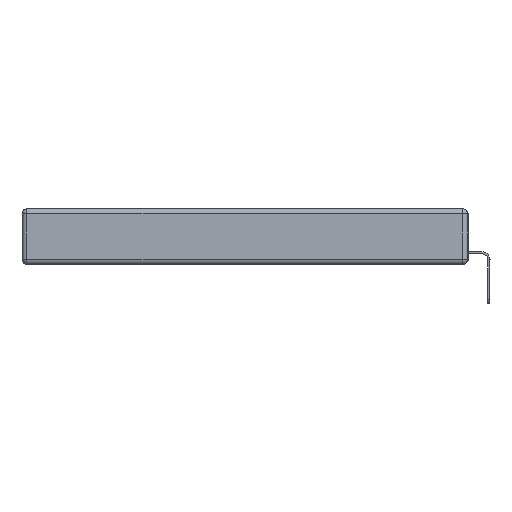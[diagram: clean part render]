
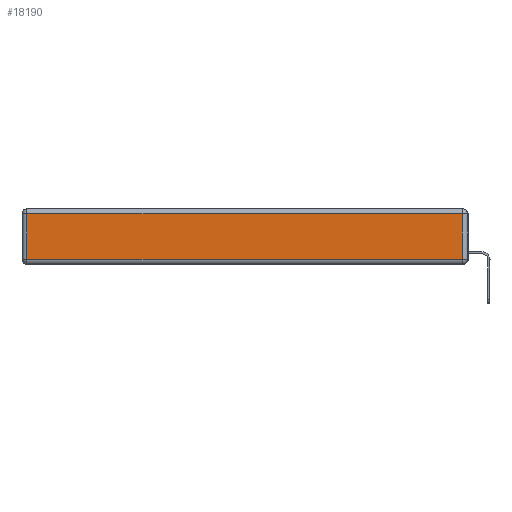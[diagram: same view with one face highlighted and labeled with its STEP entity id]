
A CAD part, left-side view. The second image highlights one B-rep face of the part: STEP entity #18190.
In plain terms, the highlighted planar face has unit normal (-1, 0, 0).
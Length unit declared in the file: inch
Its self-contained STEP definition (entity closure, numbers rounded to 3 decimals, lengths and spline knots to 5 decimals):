
#2633 = PLANE ( 'NONE',  #17909 ) ;
#3108 = DIRECTION ( 'NONE',  ( 0., 0., 1. ) ) ;
#3286 = DIRECTION ( 'NONE',  ( 0., 0., -1. ) ) ;
#3743 = VERTEX_POINT ( 'NONE', #11716 ) ;
#3861 = ORIENTED_EDGE ( 'NONE', *, *, #17575, .T. ) ;
#4161 = VERTEX_POINT ( 'NONE', #6291 ) ;
#6291 = CARTESIAN_POINT ( 'NONE',  ( 0., 2.72, -0.313 ) ) ;
#6752 = EDGE_LOOP ( 'NONE', ( #13387, #9680, #3861, #17874 ) ) ;
#8854 = VERTEX_POINT ( 'NONE', #15873 ) ;
#9680 = ORIENTED_EDGE ( 'NONE', *, *, #20982, .T. ) ;
#10116 = EDGE_CURVE ( 'NONE', #4161, #3743, #19363, .T. ) ;
#10592 = EDGE_CURVE ( 'NONE', #8854, #4161, #12771, .T. ) ;
#10761 = CARTESIAN_POINT ( 'NONE',  ( 0., 0., -0.313 ) ) ;
#11522 = VECTOR ( 'NONE', #16432, 39.37008 ) ;
#11716 = CARTESIAN_POINT ( 'NONE',  ( 0., 0.03, -0.313 ) ) ;
#12771 = LINE ( 'NONE', #13819, #17133 ) ;
#12941 = CARTESIAN_POINT ( 'NONE',  ( 0., 2.75, -0.03 ) ) ;
#13387 = ORIENTED_EDGE ( 'NONE', *, *, #10116, .T. ) ;
#13628 = CARTESIAN_POINT ( 'NONE',  ( 0., 0.03, -0.343 ) ) ;
#13819 = CARTESIAN_POINT ( 'NONE',  ( 0., 2.72, -0.343 ) ) ;
#14178 = VECTOR ( 'NONE', #19634, 39.37008 ) ;
#14919 = DIRECTION ( 'NONE',  ( 0., 0., 1. ) ) ;
#15473 = LINE ( 'NONE', #13628, #22631 ) ;
#15873 = CARTESIAN_POINT ( 'NONE',  ( 0., 2.72, -0.03 ) ) ;
#16432 = DIRECTION ( 'NONE',  ( 0., 1., 0. ) ) ;
#17133 = VECTOR ( 'NONE', #3286, 39.37008 ) ;
#17575 = EDGE_CURVE ( 'NONE', #20372, #8854, #18922, .T. ) ;
#17874 = ORIENTED_EDGE ( 'NONE', *, *, #10592, .T. ) ;
#17909 = AXIS2_PLACEMENT_3D ( 'NONE', #19955, #18330, #14919 ) ;
#18024 = FACE_OUTER_BOUND ( 'NONE', #6752, .T. ) ;
#18190 = ADVANCED_FACE ( 'NONE', ( #18024 ), #2633, .T. ) ;
#18330 = DIRECTION ( 'NONE',  ( -1., 0., 0. ) ) ;
#18922 = LINE ( 'NONE', #12941, #11522 ) ;
#19363 = LINE ( 'NONE', #10761, #14178 ) ;
#19634 = DIRECTION ( 'NONE',  ( 0., -1., 0. ) ) ;
#19955 = CARTESIAN_POINT ( 'NONE',  ( 0., 0., -0.343 ) ) ;
#20372 = VERTEX_POINT ( 'NONE', #21022 ) ;
#20982 = EDGE_CURVE ( 'NONE', #3743, #20372, #15473, .T. ) ;
#21022 = CARTESIAN_POINT ( 'NONE',  ( 0., 0.03, -0.03 ) ) ;
#22631 = VECTOR ( 'NONE', #3108, 39.37008 ) ;
